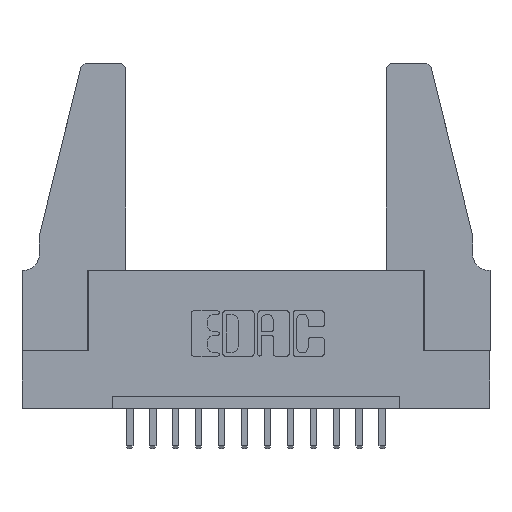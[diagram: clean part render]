
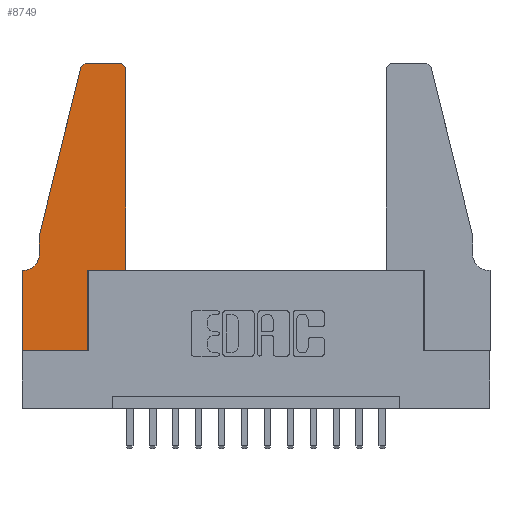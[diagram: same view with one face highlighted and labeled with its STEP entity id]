
A CAD part, top view. The second image highlights one B-rep face of the part: STEP entity #8749.
In plain terms, the highlighted planar face has unit normal (0, 0, 1).
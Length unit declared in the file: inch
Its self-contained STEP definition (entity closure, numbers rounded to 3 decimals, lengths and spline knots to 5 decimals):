
#86 = CARTESIAN_POINT ( 'NONE',  ( 0.2865, 0.35, 0.37 ) ) ;
#213 = DIRECTION ( 'NONE',  ( 0., -1., 0. ) ) ;
#252 = DIRECTION ( 'NONE',  ( 1., 0., 0. ) ) ;
#338 = ORIENTED_EDGE ( 'NONE', *, *, #5982, .T. ) ;
#578 = EDGE_LOOP ( 'NONE', ( #8951, #11432, #2966, #3407, #9312, #8146, #338, #11034, #1480, #9859, #2652, #11629 ) ) ;
#594 = DIRECTION ( 'NONE',  ( 1., 0., 0. ) ) ;
#953 = VERTEX_POINT ( 'NONE', #6216 ) ;
#1234 = LINE ( 'NONE', #2107, #13446 ) ;
#1314 = EDGE_CURVE ( 'NONE', #14705, #12073, #6639, .T. ) ;
#1389 = CARTESIAN_POINT ( 'NONE',  ( 0.2865, 0.35, 0.37 ) ) ;
#1480 = ORIENTED_EDGE ( 'NONE', *, *, #2928, .T. ) ;
#1503 = CARTESIAN_POINT ( 'NONE',  ( 0.4505, 0.35, 0.37 ) ) ;
#1539 = CARTESIAN_POINT ( 'NONE',  ( 0.0755, 0.42, 0.37 ) ) ;
#1794 = VERTEX_POINT ( 'NONE', #12056 ) ;
#1853 = CARTESIAN_POINT ( 'NONE',  ( 0.0755, 0.5, 0.37 ) ) ;
#2107 = CARTESIAN_POINT ( 'NONE',  ( 0.2605, 1.25, 0.37 ) ) ;
#2327 = CARTESIAN_POINT ( 'NONE',  ( 0.0755, 0.5, 0.37 ) ) ;
#2554 = EDGE_CURVE ( 'NONE', #9131, #15061, #7983, .T. ) ;
#2599 = CARTESIAN_POINT ( 'NONE',  ( 0.0055, 0.35, 0.37 ) ) ;
#2652 = ORIENTED_EDGE ( 'NONE', *, *, #1314, .T. ) ;
#2691 = DIRECTION ( 'NONE',  ( 0., 1., 0. ) ) ;
#2852 = VERTEX_POINT ( 'NONE', #7041 ) ;
#2928 = EDGE_CURVE ( 'NONE', #953, #3422, #9793, .T. ) ;
#2966 = ORIENTED_EDGE ( 'NONE', *, *, #10664, .T. ) ;
#3077 = DIRECTION ( 'NONE',  ( -1., 0., 0. ) ) ;
#3133 = VECTOR ( 'NONE', #2691, 39.37008 ) ;
#3325 = CIRCLE ( 'NONE', #3842, 0.03 ) ;
#3372 = CARTESIAN_POINT ( 'NONE',  ( 0.4505, 1.22, 0.37 ) ) ;
#3403 = CARTESIAN_POINT ( 'NONE',  ( 0.4205, 1.22, 0.37 ) ) ;
#3407 = ORIENTED_EDGE ( 'NONE', *, *, #10939, .T. ) ;
#3422 = VERTEX_POINT ( 'NONE', #1389 ) ;
#3550 = FACE_OUTER_BOUND ( 'NONE', #578, .T. ) ;
#3765 = LINE ( 'NONE', #4157, #6725 ) ;
#3842 = AXIS2_PLACEMENT_3D ( 'NONE', #3403, #15221, #11682 ) ;
#3966 = PLANE ( 'NONE',  #4356 ) ;
#4154 = DIRECTION ( 'NONE',  ( 0., 0., 1. ) ) ;
#4157 = CARTESIAN_POINT ( 'NONE',  ( 0.0755, 0.35, 0.37 ) ) ;
#4356 = AXIS2_PLACEMENT_3D ( 'NONE', #6288, #14574, #594 ) ;
#4474 = DIRECTION ( 'NONE',  ( -1., 0., 0. ) ) ;
#4490 = VERTEX_POINT ( 'NONE', #1539 ) ;
#4587 = CARTESIAN_POINT ( 'NONE',  ( 0.0055, 0.42, 0.37 ) ) ;
#4594 = LINE ( 'NONE', #1853, #12740 ) ;
#4760 = CARTESIAN_POINT ( 'NONE',  ( 0.4505, 0.35, 0.37 ) ) ;
#5337 = VECTOR ( 'NONE', #15031, 39.37008 ) ;
#5444 = CARTESIAN_POINT ( 'NONE',  ( 0.4505, 0.35, 0.37 ) ) ;
#5586 = EDGE_CURVE ( 'NONE', #4490, #8418, #10290, .T. ) ;
#5783 = DIRECTION ( 'NONE',  ( 0., 0., -1. ) ) ;
#5851 = CARTESIAN_POINT ( 'NONE',  ( 0., 0., 0.37 ) ) ;
#5982 = EDGE_CURVE ( 'NONE', #1794, #6479, #8611, .T. ) ;
#6216 = CARTESIAN_POINT ( 'NONE',  ( 0.2865, 0., 0.37 ) ) ;
#6288 = CARTESIAN_POINT ( 'NONE',  ( 0., 0.35, 0.37 ) ) ;
#6479 = VERTEX_POINT ( 'NONE', #5851 ) ;
#6584 = VECTOR ( 'NONE', #9383, 39.37008 ) ;
#6639 = LINE ( 'NONE', #1503, #3133 ) ;
#6641 = CARTESIAN_POINT ( 'NONE',  ( 0., 0., 0.37 ) ) ;
#6725 = VECTOR ( 'NONE', #3077, 39.37008 ) ;
#7041 = CARTESIAN_POINT ( 'NONE',  ( 0.0755, 0.5, 0.37 ) ) ;
#7358 = EDGE_CURVE ( 'NONE', #8418, #1794, #3765, .T. ) ;
#7518 = EDGE_CURVE ( 'NONE', #12073, #14840, #3325, .T. ) ;
#7706 = LINE ( 'NONE', #4760, #10454 ) ;
#7983 = CIRCLE ( 'NONE', #14669, 0.03 ) ;
#8146 = ORIENTED_EDGE ( 'NONE', *, *, #7358, .T. ) ;
#8418 = VERTEX_POINT ( 'NONE', #2599 ) ;
#8611 = LINE ( 'NONE', #14312, #6584 ) ;
#8749 = ADVANCED_FACE ( 'NONE', ( #3550 ), #3966, .T. ) ;
#8951 = ORIENTED_EDGE ( 'NONE', *, *, #12907, .T. ) ;
#9131 = VERTEX_POINT ( 'NONE', #13205 ) ;
#9312 = ORIENTED_EDGE ( 'NONE', *, *, #5586, .T. ) ;
#9367 = DIRECTION ( 'NONE',  ( -0.239, -0.971, 0. ) ) ;
#9383 = DIRECTION ( 'NONE',  ( 0., -1., 0. ) ) ;
#9446 = AXIS2_PLACEMENT_3D ( 'NONE', #4587, #5783, #15361 ) ;
#9769 = CARTESIAN_POINT ( 'NONE',  ( 0.25487, 1.22718, 0.37 ) ) ;
#9793 = LINE ( 'NONE', #86, #13134 ) ;
#9859 = ORIENTED_EDGE ( 'NONE', *, *, #13361, .T. ) ;
#10290 = CIRCLE ( 'NONE', #9446, 0.07 ) ;
#10454 = VECTOR ( 'NONE', #252, 39.37008 ) ;
#10664 = EDGE_CURVE ( 'NONE', #15061, #2852, #13302, .T. ) ;
#10939 = EDGE_CURVE ( 'NONE', #2852, #4490, #4594, .T. ) ;
#11034 = ORIENTED_EDGE ( 'NONE', *, *, #11858, .T. ) ;
#11432 = ORIENTED_EDGE ( 'NONE', *, *, #2554, .T. ) ;
#11629 = ORIENTED_EDGE ( 'NONE', *, *, #7518, .T. ) ;
#11682 = DIRECTION ( 'NONE',  ( 1., 0., 0. ) ) ;
#11858 = EDGE_CURVE ( 'NONE', #6479, #953, #14973, .T. ) ;
#12056 = CARTESIAN_POINT ( 'NONE',  ( 0., 0.35, 0.37 ) ) ;
#12073 = VERTEX_POINT ( 'NONE', #3372 ) ;
#12363 = DIRECTION ( 'NONE',  ( 1., 0., 0. ) ) ;
#12740 = VECTOR ( 'NONE', #213, 39.37008 ) ;
#12820 = CARTESIAN_POINT ( 'NONE',  ( 0.4205, 1.25, 0.37 ) ) ;
#12907 = EDGE_CURVE ( 'NONE', #14840, #9131, #1234, .T. ) ;
#13134 = VECTOR ( 'NONE', #13560, 39.37008 ) ;
#13205 = CARTESIAN_POINT ( 'NONE',  ( 0.284, 1.25, 0.37 ) ) ;
#13302 = LINE ( 'NONE', #2327, #13703 ) ;
#13361 = EDGE_CURVE ( 'NONE', #3422, #14705, #7706, .T. ) ;
#13446 = VECTOR ( 'NONE', #4474, 39.37008 ) ;
#13560 = DIRECTION ( 'NONE',  ( 0., 1., 0. ) ) ;
#13703 = VECTOR ( 'NONE', #9367, 39.37008 ) ;
#14312 = CARTESIAN_POINT ( 'NONE',  ( 0., 0., 0.37 ) ) ;
#14574 = DIRECTION ( 'NONE',  ( 0., 0., 1. ) ) ;
#14669 = AXIS2_PLACEMENT_3D ( 'NONE', #14757, #4154, #12363 ) ;
#14705 = VERTEX_POINT ( 'NONE', #5444 ) ;
#14757 = CARTESIAN_POINT ( 'NONE',  ( 0.284, 1.22, 0.37 ) ) ;
#14840 = VERTEX_POINT ( 'NONE', #12820 ) ;
#14973 = LINE ( 'NONE', #6641, #5337 ) ;
#15031 = DIRECTION ( 'NONE',  ( 1., 0., 0. ) ) ;
#15061 = VERTEX_POINT ( 'NONE', #9769 ) ;
#15221 = DIRECTION ( 'NONE',  ( 0., 0., 1. ) ) ;
#15361 = DIRECTION ( 'NONE',  ( -1., 0., 0. ) ) ;
